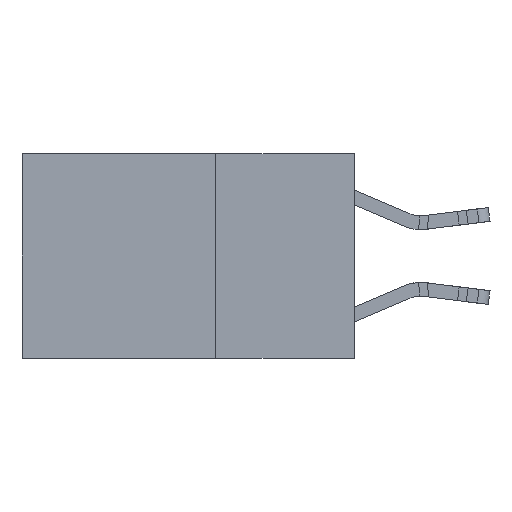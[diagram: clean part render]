
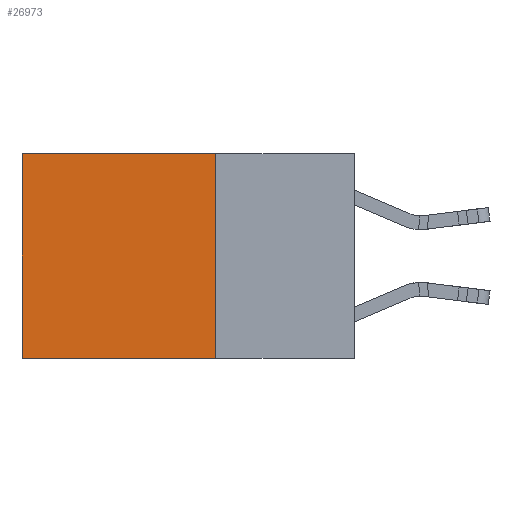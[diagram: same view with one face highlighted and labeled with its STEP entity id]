
A CAD part, left-side view. The second image highlights one B-rep face of the part: STEP entity #26973.
In plain terms, the highlighted planar face has unit normal (-1, 0, 0).
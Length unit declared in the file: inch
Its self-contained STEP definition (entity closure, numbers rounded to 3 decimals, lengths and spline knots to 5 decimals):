
#566 = VECTOR ( 'NONE', #12776, 39.37008 ) ;
#3250 = DIRECTION ( 'NONE',  ( 0., 1., 0. ) ) ;
#3316 = CARTESIAN_POINT ( 'NONE',  ( 0.2625, 0.25, 0. ) ) ;
#3583 = ORIENTED_EDGE ( 'NONE', *, *, #23877, .F. ) ;
#4011 = VERTEX_POINT ( 'NONE', #11717 ) ;
#4926 = VECTOR ( 'NONE', #30700, 39.37008 ) ;
#6526 = EDGE_CURVE ( 'NONE', #4011, #23275, #8355, .T. ) ;
#6895 = VERTEX_POINT ( 'NONE', #21942 ) ;
#6984 = DIRECTION ( 'NONE',  ( 0., 0., -1. ) ) ;
#7220 = VERTEX_POINT ( 'NONE', #26334 ) ;
#7792 = CARTESIAN_POINT ( 'NONE',  ( 0.2625, 0.25, 0. ) ) ;
#8355 = LINE ( 'NONE', #3316, #17513 ) ;
#9658 = PLANE ( 'NONE',  #23902 ) ;
#9884 = ORIENTED_EDGE ( 'NONE', *, *, #6526, .F. ) ;
#9989 = LINE ( 'NONE', #7792, #566 ) ;
#10242 = DIRECTION ( 'NONE',  ( 0., 0., -1. ) ) ;
#10335 = VECTOR ( 'NONE', #3250, 39.37008 ) ;
#11512 = LINE ( 'NONE', #21073, #4926 ) ;
#11717 = CARTESIAN_POINT ( 'NONE',  ( 0.2625, 0.25, 0. ) ) ;
#12776 = DIRECTION ( 'NONE',  ( 0., 1., 0. ) ) ;
#14977 = EDGE_LOOP ( 'NONE', ( #25595, #3583, #9884, #17577 ) ) ;
#15814 = LINE ( 'NONE', #27486, #10335 ) ;
#17459 = EDGE_CURVE ( 'NONE', #4011, #7220, #9989, .T. ) ;
#17513 = VECTOR ( 'NONE', #10242, 39.37008 ) ;
#17577 = ORIENTED_EDGE ( 'NONE', *, *, #17459, .T. ) ;
#21073 = CARTESIAN_POINT ( 'NONE',  ( 0.2625, 0.6, 0. ) ) ;
#21108 = DIRECTION ( 'NONE',  ( 1., 0., 0. ) ) ;
#21740 = FACE_OUTER_BOUND ( 'NONE', #14977, .T. ) ;
#21942 = CARTESIAN_POINT ( 'NONE',  ( 0.2625, 0.6, -0.37 ) ) ;
#23275 = VERTEX_POINT ( 'NONE', #25619 ) ;
#23877 = EDGE_CURVE ( 'NONE', #23275, #6895, #15814, .T. ) ;
#23902 = AXIS2_PLACEMENT_3D ( 'NONE', #28848, #21108, #6984 ) ;
#25595 = ORIENTED_EDGE ( 'NONE', *, *, #28830, .T. ) ;
#25619 = CARTESIAN_POINT ( 'NONE',  ( 0.2625, 0.25, -0.37 ) ) ;
#26334 = CARTESIAN_POINT ( 'NONE',  ( 0.2625, 0.6, 0. ) ) ;
#26973 = ADVANCED_FACE ( 'NONE', ( #21740 ), #9658, .F. ) ;
#27486 = CARTESIAN_POINT ( 'NONE',  ( 0.2625, 0.25, -0.37 ) ) ;
#28830 = EDGE_CURVE ( 'NONE', #7220, #6895, #11512, .T. ) ;
#28848 = CARTESIAN_POINT ( 'NONE',  ( 0.2625, 0.25, 0. ) ) ;
#30700 = DIRECTION ( 'NONE',  ( 0., 0., -1. ) ) ;
